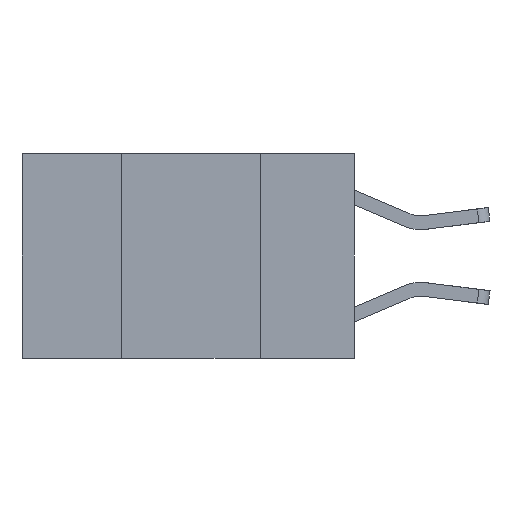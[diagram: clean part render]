
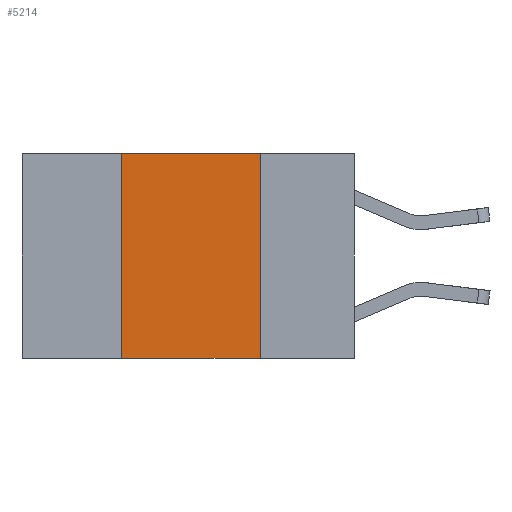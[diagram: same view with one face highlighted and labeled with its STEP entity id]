
A CAD part, left-side view. The second image highlights one B-rep face of the part: STEP entity #5214.
In plain terms, the highlighted planar face has unit normal (-1, 0, 0).
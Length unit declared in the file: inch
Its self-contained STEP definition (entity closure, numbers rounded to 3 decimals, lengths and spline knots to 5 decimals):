
#649 = ORIENTED_EDGE ( 'NONE', *, *, #4689, .F. ) ;
#833 = FACE_OUTER_BOUND ( 'NONE', #4455, .T. ) ;
#840 = PLANE ( 'NONE',  #1674 ) ;
#1512 = LINE ( 'NONE', #5087, #3768 ) ;
#1516 = CARTESIAN_POINT ( 'NONE',  ( 0., 0.6, -0.37 ) ) ;
#1674 = AXIS2_PLACEMENT_3D ( 'NONE', #2537, #8442, #3406 ) ;
#2022 = VERTEX_POINT ( 'NONE', #4842 ) ;
#2537 = CARTESIAN_POINT ( 'NONE',  ( 0., 0.6, 0. ) ) ;
#2720 = VERTEX_POINT ( 'NONE', #9190 ) ;
#2778 = EDGE_CURVE ( 'NONE', #2022, #2720, #1512, .T. ) ;
#3225 = EDGE_CURVE ( 'NONE', #2022, #10800, #10475, .T. ) ;
#3288 = CARTESIAN_POINT ( 'NONE',  ( 0., 0.17, -0.37 ) ) ;
#3316 = VERTEX_POINT ( 'NONE', #8404 ) ;
#3341 = LINE ( 'NONE', #10005, #5325 ) ;
#3406 = DIRECTION ( 'NONE',  ( 0., 0., -1. ) ) ;
#3768 = VECTOR ( 'NONE', #10943, 39.37008 ) ;
#4365 = DIRECTION ( 'NONE',  ( 0., -1., 0. ) ) ;
#4455 = EDGE_LOOP ( 'NONE', ( #7146, #649, #5167, #7418 ) ) ;
#4493 = EDGE_CURVE ( 'NONE', #3316, #10800, #3341, .T. ) ;
#4689 = EDGE_CURVE ( 'NONE', #2720, #3316, #5996, .T. ) ;
#4842 = CARTESIAN_POINT ( 'NONE',  ( 0., 0.42, -0.37 ) ) ;
#5087 = CARTESIAN_POINT ( 'NONE',  ( 0., 0.42, 0. ) ) ;
#5167 = ORIENTED_EDGE ( 'NONE', *, *, #2778, .F. ) ;
#5214 = ADVANCED_FACE ( 'NONE', ( #833 ), #840, .F. ) ;
#5325 = VECTOR ( 'NONE', #10845, 39.37008 ) ;
#5996 = LINE ( 'NONE', #9364, #9922 ) ;
#6026 = VECTOR ( 'NONE', #7441, 39.37008 ) ;
#7146 = ORIENTED_EDGE ( 'NONE', *, *, #4493, .F. ) ;
#7418 = ORIENTED_EDGE ( 'NONE', *, *, #3225, .T. ) ;
#7441 = DIRECTION ( 'NONE',  ( 0., -1., 0. ) ) ;
#8404 = CARTESIAN_POINT ( 'NONE',  ( 0., 0.17, 0. ) ) ;
#8442 = DIRECTION ( 'NONE',  ( 1., 0., 0. ) ) ;
#9190 = CARTESIAN_POINT ( 'NONE',  ( 0., 0.42, 0. ) ) ;
#9364 = CARTESIAN_POINT ( 'NONE',  ( 0., 0.6, 0. ) ) ;
#9922 = VECTOR ( 'NONE', #4365, 39.37008 ) ;
#10005 = CARTESIAN_POINT ( 'NONE',  ( 0., 0.17, 0. ) ) ;
#10475 = LINE ( 'NONE', #1516, #6026 ) ;
#10800 = VERTEX_POINT ( 'NONE', #3288 ) ;
#10845 = DIRECTION ( 'NONE',  ( 0., 0., -1. ) ) ;
#10943 = DIRECTION ( 'NONE',  ( 0., 0., 1. ) ) ;
